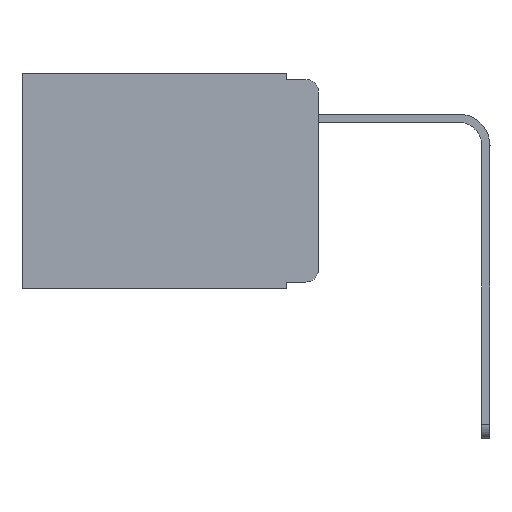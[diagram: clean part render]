
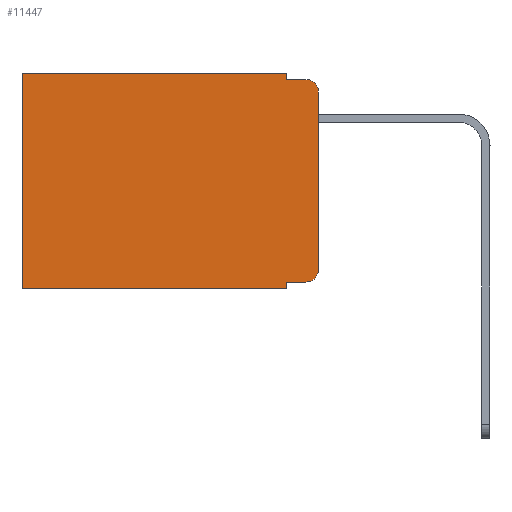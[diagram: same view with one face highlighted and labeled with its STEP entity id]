
A CAD part, left-side view. The second image highlights one B-rep face of the part: STEP entity #11447.
In plain terms, the highlighted planar face has unit normal (-1, 0, 0).
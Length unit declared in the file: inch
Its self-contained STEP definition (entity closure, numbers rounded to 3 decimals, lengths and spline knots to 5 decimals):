
#96 = DIRECTION ( 'NONE',  ( 0., 0., -1. ) ) ;
#196 = CARTESIAN_POINT ( 'NONE',  ( 0.298, 0., 0. ) ) ;
#408 = DIRECTION ( 'NONE',  ( 0., 0., -1. ) ) ;
#411 = CARTESIAN_POINT ( 'NONE',  ( 0.298, 0.02, -0.313 ) ) ;
#503 = CARTESIAN_POINT ( 'NONE',  ( 0.298, 0., 0. ) ) ;
#794 = VERTEX_POINT ( 'NONE', #11300 ) ;
#871 = FACE_OUTER_BOUND ( 'NONE', #4650, .T. ) ;
#877 = ORIENTED_EDGE ( 'NONE', *, *, #2714, .F. ) ;
#880 = EDGE_CURVE ( 'NONE', #5889, #11106, #9038, .T. ) ;
#1215 = EDGE_CURVE ( 'NONE', #3318, #11888, #12027, .T. ) ;
#1228 = CARTESIAN_POINT ( 'NONE',  ( 0.298, 0.051, 0. ) ) ;
#1238 = EDGE_CURVE ( 'NONE', #11106, #11888, #8883, .T. ) ;
#1324 = CARTESIAN_POINT ( 'NONE',  ( 0.298, 0., -0.343 ) ) ;
#1556 = CARTESIAN_POINT ( 'NONE',  ( 0.298, 0.02, -0.01 ) ) ;
#1586 = LINE ( 'NONE', #9400, #7287 ) ;
#1744 = EDGE_CURVE ( 'NONE', #794, #5319, #4122, .T. ) ;
#1787 = CARTESIAN_POINT ( 'NONE',  ( 0.298, 0.473, 0. ) ) ;
#1976 = LINE ( 'NONE', #11682, #2126 ) ;
#2064 = ORIENTED_EDGE ( 'NONE', *, *, #11177, .F. ) ;
#2126 = VECTOR ( 'NONE', #7016, 39.37008 ) ;
#2212 = CARTESIAN_POINT ( 'NONE',  ( 0.298, 0., -0.313 ) ) ;
#2283 = DIRECTION ( 'NONE',  ( -1., 0., 0. ) ) ;
#2377 = VERTEX_POINT ( 'NONE', #1556 ) ;
#2522 = VERTEX_POINT ( 'NONE', #9824 ) ;
#2696 = DIRECTION ( 'NONE',  ( 0., -1., 0. ) ) ;
#2714 = EDGE_CURVE ( 'NONE', #5889, #2522, #1976, .T. ) ;
#2790 = VERTEX_POINT ( 'NONE', #5160 ) ;
#3114 = VECTOR ( 'NONE', #8831, 39.37008 ) ;
#3263 = VECTOR ( 'NONE', #408, 39.37008 ) ;
#3301 = DIRECTION ( 'NONE',  ( 0., 0., -1. ) ) ;
#3318 = VERTEX_POINT ( 'NONE', #6119 ) ;
#3508 = DIRECTION ( 'NONE',  ( 0., 0., -1. ) ) ;
#3689 = DIRECTION ( 'NONE',  ( 0., -1., 0. ) ) ;
#4042 = VECTOR ( 'NONE', #8228, 39.37008 ) ;
#4122 = LINE ( 'NONE', #1228, #7860 ) ;
#4157 = AXIS2_PLACEMENT_3D ( 'NONE', #7323, #4404, #3508 ) ;
#4174 = AXIS2_PLACEMENT_3D ( 'NONE', #411, #2283, #3301 ) ;
#4196 = CARTESIAN_POINT ( 'NONE',  ( 0.298, 0.02, -0.333 ) ) ;
#4238 = ORIENTED_EDGE ( 'NONE', *, *, #11275, .T. ) ;
#4404 = DIRECTION ( 'NONE',  ( -1., 0., 0. ) ) ;
#4531 = CARTESIAN_POINT ( 'NONE',  ( 0.298, 0.051, -0.333 ) ) ;
#4650 = EDGE_LOOP ( 'NONE', ( #12331, #11631, #9659, #9665, #7256, #4238, #2064, #877, #7995, #8868 ) ) ;
#4753 = VECTOR ( 'NONE', #2696, 39.37008 ) ;
#4788 = LINE ( 'NONE', #8956, #3114 ) ;
#4947 = PLANE ( 'NONE',  #11762 ) ;
#5008 = DIRECTION ( 'NONE',  ( 0., 0., -1. ) ) ;
#5160 = CARTESIAN_POINT ( 'NONE',  ( 0.298, 0.473, -0.343 ) ) ;
#5319 = VERTEX_POINT ( 'NONE', #6311 ) ;
#5468 = VERTEX_POINT ( 'NONE', #1787 ) ;
#5889 = VERTEX_POINT ( 'NONE', #4531 ) ;
#6119 = CARTESIAN_POINT ( 'NONE',  ( 0.298, 0., -0.03 ) ) ;
#6311 = CARTESIAN_POINT ( 'NONE',  ( 0.298, 0.051, -0.01 ) ) ;
#7016 = DIRECTION ( 'NONE',  ( 0., 0., -1. ) ) ;
#7256 = ORIENTED_EDGE ( 'NONE', *, *, #11575, .T. ) ;
#7287 = VECTOR ( 'NONE', #3689, 39.37008 ) ;
#7323 = CARTESIAN_POINT ( 'NONE',  ( 0.298, 0.02, -0.03 ) ) ;
#7707 = DIRECTION ( 'NONE',  ( 1., 0., 0. ) ) ;
#7860 = VECTOR ( 'NONE', #5008, 39.37008 ) ;
#7995 = ORIENTED_EDGE ( 'NONE', *, *, #880, .T. ) ;
#8148 = EDGE_CURVE ( 'NONE', #3318, #2377, #10576, .T. ) ;
#8228 = DIRECTION ( 'NONE',  ( 0., 1., 0. ) ) ;
#8831 = DIRECTION ( 'NONE',  ( 0., 1., 0. ) ) ;
#8868 = ORIENTED_EDGE ( 'NONE', *, *, #1238, .T. ) ;
#8883 = CIRCLE ( 'NONE', #4174, 0.02 ) ;
#8956 = CARTESIAN_POINT ( 'NONE',  ( 0.298, 0., 0. ) ) ;
#9038 = LINE ( 'NONE', #12236, #4753 ) ;
#9051 = CARTESIAN_POINT ( 'NONE',  ( 0.298, 0.473, 0. ) ) ;
#9400 = CARTESIAN_POINT ( 'NONE',  ( 0.298, 0.051, -0.01 ) ) ;
#9641 = DIRECTION ( 'NONE',  ( 0., 0., -1. ) ) ;
#9659 = ORIENTED_EDGE ( 'NONE', *, *, #12246, .F. ) ;
#9665 = ORIENTED_EDGE ( 'NONE', *, *, #1744, .F. ) ;
#9824 = CARTESIAN_POINT ( 'NONE',  ( 0.298, 0.051, -0.343 ) ) ;
#9934 = VECTOR ( 'NONE', #96, 39.37008 ) ;
#10140 = LINE ( 'NONE', #1324, #4042 ) ;
#10576 = CIRCLE ( 'NONE', #4157, 0.02 ) ;
#10731 = LINE ( 'NONE', #9051, #3263 ) ;
#11106 = VERTEX_POINT ( 'NONE', #4196 ) ;
#11177 = EDGE_CURVE ( 'NONE', #2522, #2790, #10140, .T. ) ;
#11275 = EDGE_CURVE ( 'NONE', #5468, #2790, #10731, .T. ) ;
#11300 = CARTESIAN_POINT ( 'NONE',  ( 0.298, 0.051, 0. ) ) ;
#11447 = ADVANCED_FACE ( 'NONE', ( #871 ), #4947, .F. ) ;
#11575 = EDGE_CURVE ( 'NONE', #794, #5468, #4788, .T. ) ;
#11631 = ORIENTED_EDGE ( 'NONE', *, *, #8148, .T. ) ;
#11682 = CARTESIAN_POINT ( 'NONE',  ( 0.298, 0.051, 0. ) ) ;
#11762 = AXIS2_PLACEMENT_3D ( 'NONE', #196, #7707, #9641 ) ;
#11888 = VERTEX_POINT ( 'NONE', #2212 ) ;
#12027 = LINE ( 'NONE', #503, #9934 ) ;
#12236 = CARTESIAN_POINT ( 'NONE',  ( 0.298, 0.051, -0.333 ) ) ;
#12246 = EDGE_CURVE ( 'NONE', #5319, #2377, #1586, .T. ) ;
#12331 = ORIENTED_EDGE ( 'NONE', *, *, #1215, .F. ) ;
